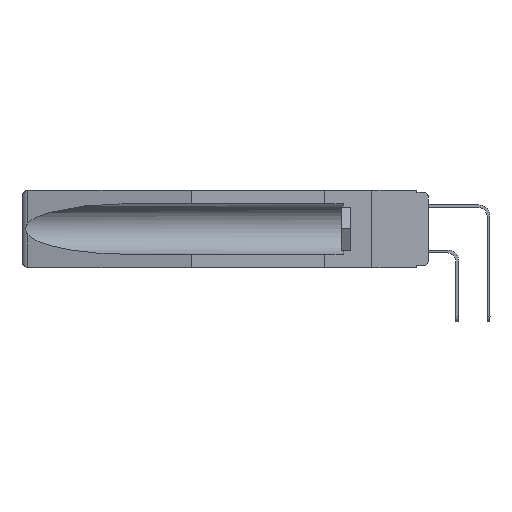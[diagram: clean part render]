
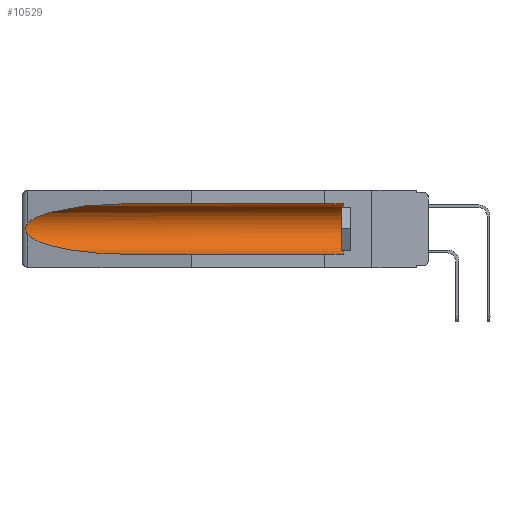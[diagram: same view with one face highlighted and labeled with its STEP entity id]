
A CAD part, left-side view. The second image highlights one B-rep face of the part: STEP entity #10529.
In plain terms, the highlighted cylindrical face has radius 2.857 mm (diameter 5.715 mm), a partial arc.
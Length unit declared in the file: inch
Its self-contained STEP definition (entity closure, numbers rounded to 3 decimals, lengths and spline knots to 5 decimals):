
#296 = CARTESIAN_POINT ( 'NONE',  ( 0.155, 1.07973, -0.284 ) ) ;
#749 =( BOUNDED_CURVE ( )  B_SPLINE_CURVE ( 3, ( #5684, #9550, #5423, #15173 ),
 .UNSPECIFIED., .F., .T. ) 
 B_SPLINE_CURVE_WITH_KNOTS ( ( 4, 4 ),
 ( 4.71239, 6.08839 ),
 .UNSPECIFIED. ) 
 CURVE ( )  GEOMETRIC_REPRESENTATION_ITEM ( )  RATIONAL_B_SPLINE_CURVE ( ( 1., 0.848, 0.848, 1. ) ) 
 REPRESENTATION_ITEM ( '' )  );
#780 = EDGE_CURVE ( 'NONE', #11487, #24035, #13223, .T. ) ;
#807 = EDGE_CURVE ( 'NONE', #13355, #8147, #12493, .T. ) ;
#1502 = VERTEX_POINT ( 'NONE', #19990 ) ;
#1989 = CARTESIAN_POINT ( 'NONE',  ( 0.26597, 1.52961, -0.15275 ) ) ;
#3619 = EDGE_LOOP ( 'NONE', ( #7933, #15701, #21372, #10787, #20442, #15897 ) ) ;
#3636 = CARTESIAN_POINT ( 'NONE',  ( 0.26655, 1.53094, -0.18657 ) ) ;
#3687 = AXIS2_PLACEMENT_3D ( 'NONE', #22955, #13389, #16954 ) ;
#4004 = CARTESIAN_POINT ( 'NONE',  ( 0.26654, 1.53092, -0.15636 ) ) ;
#4201 = CARTESIAN_POINT ( 'NONE',  ( 0.21114, 1.30732, -0.284 ) ) ;
#5029 = AXIS2_PLACEMENT_3D ( 'NONE', #13373, #15538, #19498 ) ;
#5423 = CARTESIAN_POINT ( 'NONE',  ( 0.25451, 1.48313, -0.09465 ) ) ;
#5671 = CARTESIAN_POINT ( 'NONE',  ( 0.26597, 1.5296, -0.19026 ) ) ;
#5684 = CARTESIAN_POINT ( 'NONE',  ( 0.155, 1.07973, -0.059 ) ) ;
#5920 = CARTESIAN_POINT ( 'NONE',  ( 0.2675, 1.53308, -0.17534 ) ) ;
#7894 = EDGE_CURVE ( 'NONE', #11487, #1502, #17945, .T. ) ;
#7933 = ORIENTED_EDGE ( 'NONE', *, *, #9417, .T. ) ;
#7967 = CARTESIAN_POINT ( 'NONE',  ( 0.2673, 1.53269, -0.17917 ) ) ;
#8022 = EDGE_CURVE ( 'NONE', #24035, #16245, #12972, .T. ) ;
#8147 = VERTEX_POINT ( 'NONE', #23281 ) ;
#8490 = DIRECTION ( 'NONE',  ( 0., 1., 0. ) ) ;
#8750 = EDGE_CURVE ( 'NONE', #8147, #1502, #8851, .T. ) ;
#8851 =( BOUNDED_CURVE ( )  B_SPLINE_CURVE ( 3, ( #23739, #17759, #4201, #296 ),
 .UNSPECIFIED., .F., .F. ) 
 B_SPLINE_CURVE_WITH_KNOTS ( ( 4, 4 ),
 ( 0.1948, 1.5708 ),
 .UNSPECIFIED. ) 
 CURVE ( )  GEOMETRIC_REPRESENTATION_ITEM ( )  RATIONAL_B_SPLINE_CURVE ( ( 1., 0.848, 0.848, 1. ) ) 
 REPRESENTATION_ITEM ( '' )  );
#8862 = CARTESIAN_POINT ( 'NONE',  ( 0.155, -0.30754, -0.059 ) ) ;
#9417 = EDGE_CURVE ( 'NONE', #16245, #13355, #749, .T. ) ;
#9550 = CARTESIAN_POINT ( 'NONE',  ( 0.21114, 1.30732, -0.059 ) ) ;
#10066 = CARTESIAN_POINT ( 'NONE',  ( 0.155, 0.126, -0.059 ) ) ;
#10529 = ADVANCED_FACE ( 'NONE', ( #15298 ), #24727, .F. ) ;
#10787 = ORIENTED_EDGE ( 'NONE', *, *, #7894, .F. ) ;
#11346 = VECTOR ( 'NONE', #24435, 39.37008 ) ;
#11449 = CARTESIAN_POINT ( 'NONE',  ( 0.26537, 1.52718, -0.19328 ) ) ;
#11487 = VERTEX_POINT ( 'NONE', #20329 ) ;
#12493 = B_SPLINE_CURVE_WITH_KNOTS ( 'NONE', 3,
 ( #25093, #1989, #4004, #17326, #23310, #5920, #7967, #3636, #5671, #11449 ),
 .UNSPECIFIED., .F., .F.,
 ( 4, 2, 2, 2, 4 ),
 ( 0., 0.00029, 0.00058, 0.00087, 0.00117 ),
 .UNSPECIFIED. ) ;
#12972 = LINE ( 'NONE', #8862, #11346 ) ;
#12986 = VECTOR ( 'NONE', #8490, 39.37008 ) ;
#13223 = CIRCLE ( 'NONE', #5029, 0.1125 ) ;
#13355 = VERTEX_POINT ( 'NONE', #17092 ) ;
#13373 = CARTESIAN_POINT ( 'NONE',  ( 0.155, 0.126, -0.1715 ) ) ;
#13389 = DIRECTION ( 'NONE',  ( 0., 1., 0. ) ) ;
#15173 = CARTESIAN_POINT ( 'NONE',  ( 0.26537, 1.52718, -0.14972 ) ) ;
#15298 = FACE_OUTER_BOUND ( 'NONE', #3619, .T. ) ;
#15538 = DIRECTION ( 'NONE',  ( 0., -1., 0. ) ) ;
#15701 = ORIENTED_EDGE ( 'NONE', *, *, #807, .T. ) ;
#15897 = ORIENTED_EDGE ( 'NONE', *, *, #8022, .T. ) ;
#16041 = CARTESIAN_POINT ( 'NONE',  ( 0.155, -0.30754, -0.284 ) ) ;
#16245 = VERTEX_POINT ( 'NONE', #16360 ) ;
#16360 = CARTESIAN_POINT ( 'NONE',  ( 0.155, 1.07973, -0.059 ) ) ;
#16954 = DIRECTION ( 'NONE',  ( 0., 0., 1. ) ) ;
#17092 = CARTESIAN_POINT ( 'NONE',  ( 0.26537, 1.52718, -0.14972 ) ) ;
#17326 = CARTESIAN_POINT ( 'NONE',  ( 0.2673, 1.5327, -0.16383 ) ) ;
#17759 = CARTESIAN_POINT ( 'NONE',  ( 0.25451, 1.48313, -0.24835 ) ) ;
#17945 = LINE ( 'NONE', #16041, #12986 ) ;
#19498 = DIRECTION ( 'NONE',  ( 0., 0., 1. ) ) ;
#19990 = CARTESIAN_POINT ( 'NONE',  ( 0.155, 1.07973, -0.284 ) ) ;
#20329 = CARTESIAN_POINT ( 'NONE',  ( 0.155, 0.126, -0.284 ) ) ;
#20442 = ORIENTED_EDGE ( 'NONE', *, *, #780, .T. ) ;
#21372 = ORIENTED_EDGE ( 'NONE', *, *, #8750, .T. ) ;
#22955 = CARTESIAN_POINT ( 'NONE',  ( 0.155, -0.30754, -0.1715 ) ) ;
#23281 = CARTESIAN_POINT ( 'NONE',  ( 0.26537, 1.52718, -0.19328 ) ) ;
#23310 = CARTESIAN_POINT ( 'NONE',  ( 0.2675, 1.53308, -0.16763 ) ) ;
#23739 = CARTESIAN_POINT ( 'NONE',  ( 0.26537, 1.52718, -0.19328 ) ) ;
#24035 = VERTEX_POINT ( 'NONE', #10066 ) ;
#24435 = DIRECTION ( 'NONE',  ( 0., 1., 0. ) ) ;
#24727 = CYLINDRICAL_SURFACE ( 'NONE', #3687, 0.1125 ) ;
#25093 = CARTESIAN_POINT ( 'NONE',  ( 0.26537, 1.52718, -0.14972 ) ) ;
